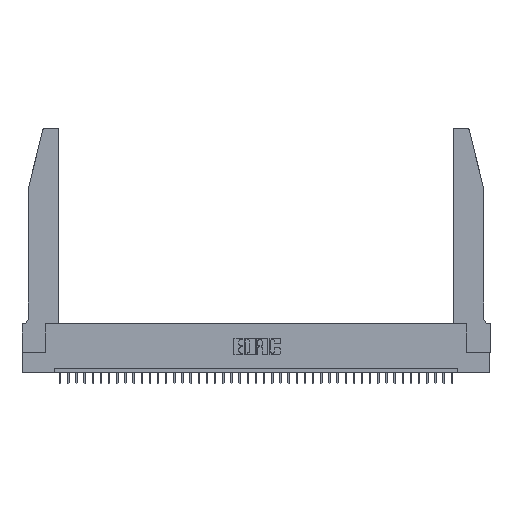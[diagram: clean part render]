
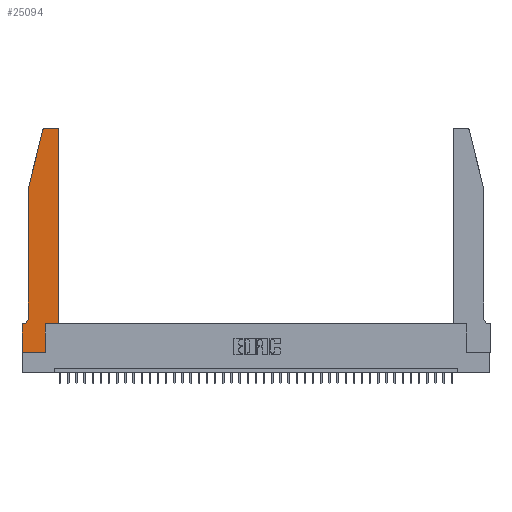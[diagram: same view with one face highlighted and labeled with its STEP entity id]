
A CAD part, top view. The second image highlights one B-rep face of the part: STEP entity #25094.
In plain terms, the highlighted planar face has unit normal (0, 0, 1).
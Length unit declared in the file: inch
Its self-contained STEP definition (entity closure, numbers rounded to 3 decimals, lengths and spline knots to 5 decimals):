
#1874 = CARTESIAN_POINT ( 'NONE',  ( 0.0755, 0.35, 0.37 ) ) ;
#2076 = DIRECTION ( 'NONE',  ( -1., 0., 0. ) ) ;
#2112 = CARTESIAN_POINT ( 'NONE',  ( 0.2865, 0.35, 0.37 ) ) ;
#2314 = LINE ( 'NONE', #13677, #32576 ) ;
#2801 = EDGE_CURVE ( 'NONE', #26073, #27545, #33669, .T. ) ;
#2894 = CARTESIAN_POINT ( 'NONE',  ( 0.0755, 0.42, 0.37 ) ) ;
#3088 = VERTEX_POINT ( 'NONE', #30359 ) ;
#3340 = CIRCLE ( 'NONE', #12539, 0.07 ) ;
#3809 = EDGE_CURVE ( 'NONE', #3088, #40105, #2314, .T. ) ;
#4193 = ORIENTED_EDGE ( 'NONE', *, *, #26312, .T. ) ;
#5213 = LINE ( 'NONE', #2112, #22908 ) ;
#5846 = DIRECTION ( 'NONE',  ( 0., 0., -1. ) ) ;
#6613 = ORIENTED_EDGE ( 'NONE', *, *, #10118, .T. ) ;
#6671 = VERTEX_POINT ( 'NONE', #14338 ) ;
#6857 = EDGE_CURVE ( 'NONE', #23194, #9921, #22805, .T. ) ;
#6978 = CARTESIAN_POINT ( 'NONE',  ( 0., 0., 0.37 ) ) ;
#7038 = ORIENTED_EDGE ( 'NONE', *, *, #10795, .T. ) ;
#7178 = CARTESIAN_POINT ( 'NONE',  ( 0.2865, 0., 0.37 ) ) ;
#7682 = CARTESIAN_POINT ( 'NONE',  ( 0.284, 2.75, 0.37 ) ) ;
#8254 = VERTEX_POINT ( 'NONE', #27905 ) ;
#8400 = DIRECTION ( 'NONE',  ( 1., 0., 0. ) ) ;
#8752 = CARTESIAN_POINT ( 'NONE',  ( 0.4205, 2.75, 0.37 ) ) ;
#9013 = CARTESIAN_POINT ( 'NONE',  ( 0.0755, 2., 0.37 ) ) ;
#9231 = ORIENTED_EDGE ( 'NONE', *, *, #10984, .T. ) ;
#9921 = VERTEX_POINT ( 'NONE', #7178 ) ;
#10118 = EDGE_CURVE ( 'NONE', #27545, #33398, #31507, .T. ) ;
#10164 = DIRECTION ( 'NONE',  ( 1., 0., 0. ) ) ;
#10472 = VECTOR ( 'NONE', #12735, 39.37008 ) ;
#10795 = EDGE_CURVE ( 'NONE', #9921, #24922, #5213, .T. ) ;
#10935 = FACE_OUTER_BOUND ( 'NONE', #21591, .T. ) ;
#10984 = EDGE_CURVE ( 'NONE', #23066, #23194, #34487, .T. ) ;
#11603 = DIRECTION ( 'NONE',  ( 0., 1., 0. ) ) ;
#11820 = DIRECTION ( 'NONE',  ( -1., 0., 0. ) ) ;
#11823 = CARTESIAN_POINT ( 'NONE',  ( 0.4205, 2.72, 0.37 ) ) ;
#12474 = EDGE_CURVE ( 'NONE', #24922, #3088, #33215, .T. ) ;
#12539 = AXIS2_PLACEMENT_3D ( 'NONE', #30622, #5846, #11820 ) ;
#12735 = DIRECTION ( 'NONE',  ( -0.239, -0.971, 0. ) ) ;
#13677 = CARTESIAN_POINT ( 'NONE',  ( 0.4505, 0.35, 0.37 ) ) ;
#14338 = CARTESIAN_POINT ( 'NONE',  ( 0.0755, 2., 0.37 ) ) ;
#16545 = DIRECTION ( 'NONE',  ( 0., -1., 0. ) ) ;
#17027 = LINE ( 'NONE', #32678, #26453 ) ;
#18658 = ORIENTED_EDGE ( 'NONE', *, *, #36218, .T. ) ;
#19024 = AXIS2_PLACEMENT_3D ( 'NONE', #27660, #40177, #8400 ) ;
#20273 = VECTOR ( 'NONE', #16545, 39.37008 ) ;
#20733 = DIRECTION ( 'NONE',  ( 0., -1., 0. ) ) ;
#21561 = CARTESIAN_POINT ( 'NONE',  ( 0., 0., 0.37 ) ) ;
#21591 = EDGE_LOOP ( 'NONE', ( #30926, #6613, #25253, #4193, #18658, #31860, #9231, #36538, #7038, #28858, #24094, #26926 ) ) ;
#22805 = LINE ( 'NONE', #39059, #30655 ) ;
#22908 = VECTOR ( 'NONE', #11603, 39.37008 ) ;
#23066 = VERTEX_POINT ( 'NONE', #33109 ) ;
#23101 = EDGE_CURVE ( 'NONE', #40105, #26073, #30197, .T. ) ;
#23194 = VERTEX_POINT ( 'NONE', #21561 ) ;
#23992 = DIRECTION ( 'NONE',  ( -1., 0., 0. ) ) ;
#24094 = ORIENTED_EDGE ( 'NONE', *, *, #3809, .T. ) ;
#24406 = CARTESIAN_POINT ( 'NONE',  ( 0.2605, 2.75, 0.37 ) ) ;
#24702 = CARTESIAN_POINT ( 'NONE',  ( 0.25487, 2.72718, 0.37 ) ) ;
#24760 = LINE ( 'NONE', #9013, #10472 ) ;
#24922 = VERTEX_POINT ( 'NONE', #31215 ) ;
#25094 = ADVANCED_FACE ( 'NONE', ( #10935 ), #25866, .T. ) ;
#25253 = ORIENTED_EDGE ( 'NONE', *, *, #34728, .T. ) ;
#25326 = VERTEX_POINT ( 'NONE', #2894 ) ;
#25866 = PLANE ( 'NONE',  #30310 ) ;
#26073 = VERTEX_POINT ( 'NONE', #8752 ) ;
#26275 = CARTESIAN_POINT ( 'NONE',  ( 0., 0.35, 0.37 ) ) ;
#26312 = EDGE_CURVE ( 'NONE', #6671, #25326, #17027, .T. ) ;
#26453 = VECTOR ( 'NONE', #20733, 39.37008 ) ;
#26456 = CARTESIAN_POINT ( 'NONE',  ( 0.4505, 0.35, 0.37 ) ) ;
#26926 = ORIENTED_EDGE ( 'NONE', *, *, #23101, .T. ) ;
#26956 = DIRECTION ( 'NONE',  ( 1., 0., 0. ) ) ;
#27545 = VERTEX_POINT ( 'NONE', #7682 ) ;
#27623 = VECTOR ( 'NONE', #38592, 39.37008 ) ;
#27660 = CARTESIAN_POINT ( 'NONE',  ( 0.284, 2.72, 0.37 ) ) ;
#27905 = CARTESIAN_POINT ( 'NONE',  ( 0.0055, 0.35, 0.37 ) ) ;
#28858 = ORIENTED_EDGE ( 'NONE', *, *, #12474, .T. ) ;
#30175 = LINE ( 'NONE', #1874, #38612 ) ;
#30179 = DIRECTION ( 'NONE',  ( 0., 1., 0. ) ) ;
#30197 = CIRCLE ( 'NONE', #32172, 0.03 ) ;
#30232 = DIRECTION ( 'NONE',  ( 0., 0., 1. ) ) ;
#30310 = AXIS2_PLACEMENT_3D ( 'NONE', #26275, #39014, #39217 ) ;
#30359 = CARTESIAN_POINT ( 'NONE',  ( 0.4505, 0.35, 0.37 ) ) ;
#30622 = CARTESIAN_POINT ( 'NONE',  ( 0.0055, 0.42, 0.37 ) ) ;
#30655 = VECTOR ( 'NONE', #10164, 39.37008 ) ;
#30926 = ORIENTED_EDGE ( 'NONE', *, *, #2801, .T. ) ;
#30931 = EDGE_CURVE ( 'NONE', #8254, #23066, #30175, .T. ) ;
#31215 = CARTESIAN_POINT ( 'NONE',  ( 0.2865, 0.35, 0.37 ) ) ;
#31507 = CIRCLE ( 'NONE', #19024, 0.03 ) ;
#31860 = ORIENTED_EDGE ( 'NONE', *, *, #30931, .T. ) ;
#32172 = AXIS2_PLACEMENT_3D ( 'NONE', #11823, #30232, #26956 ) ;
#32576 = VECTOR ( 'NONE', #30179, 39.37008 ) ;
#32678 = CARTESIAN_POINT ( 'NONE',  ( 0.0755, 2., 0.37 ) ) ;
#33109 = CARTESIAN_POINT ( 'NONE',  ( 0., 0.35, 0.37 ) ) ;
#33215 = LINE ( 'NONE', #26456, #27623 ) ;
#33398 = VERTEX_POINT ( 'NONE', #24702 ) ;
#33669 = LINE ( 'NONE', #24406, #34020 ) ;
#34020 = VECTOR ( 'NONE', #23992, 39.37008 ) ;
#34206 = CARTESIAN_POINT ( 'NONE',  ( 0.4505, 2.72, 0.37 ) ) ;
#34487 = LINE ( 'NONE', #6978, #20273 ) ;
#34728 = EDGE_CURVE ( 'NONE', #33398, #6671, #24760, .T. ) ;
#36218 = EDGE_CURVE ( 'NONE', #25326, #8254, #3340, .T. ) ;
#36538 = ORIENTED_EDGE ( 'NONE', *, *, #6857, .T. ) ;
#38592 = DIRECTION ( 'NONE',  ( 1., 0., 0. ) ) ;
#38612 = VECTOR ( 'NONE', #2076, 39.37008 ) ;
#39014 = DIRECTION ( 'NONE',  ( 0., 0., 1. ) ) ;
#39059 = CARTESIAN_POINT ( 'NONE',  ( 0., 0., 0.37 ) ) ;
#39217 = DIRECTION ( 'NONE',  ( 1., 0., 0. ) ) ;
#40105 = VERTEX_POINT ( 'NONE', #34206 ) ;
#40177 = DIRECTION ( 'NONE',  ( 0., 0., 1. ) ) ;
